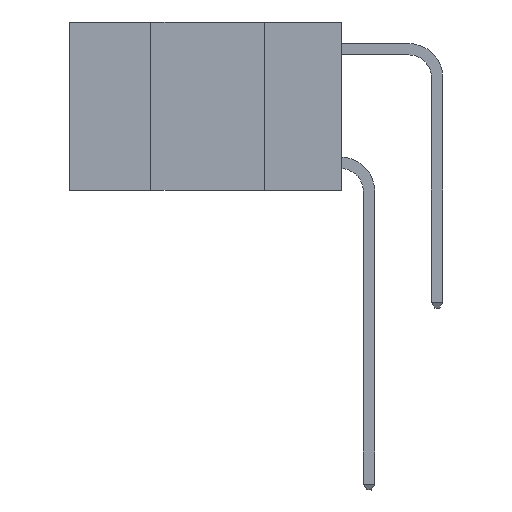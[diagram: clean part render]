
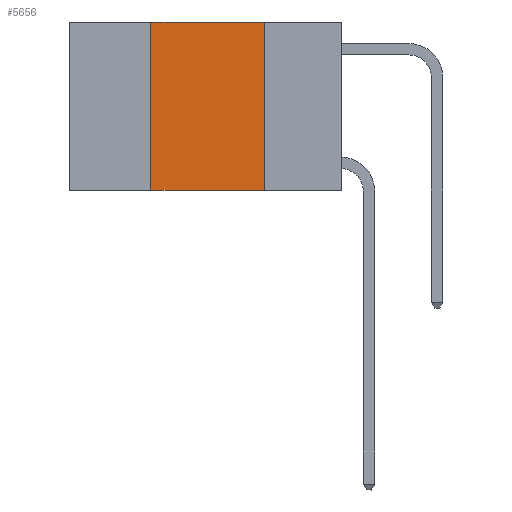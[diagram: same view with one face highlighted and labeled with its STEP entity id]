
A CAD part, left-side view. The second image highlights one B-rep face of the part: STEP entity #5656.
In plain terms, the highlighted planar face has unit normal (-1, 0, 0).
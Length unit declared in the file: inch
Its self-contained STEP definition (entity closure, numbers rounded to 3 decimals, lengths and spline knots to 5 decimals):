
#316 = FACE_OUTER_BOUND ( 'NONE', #9335, .T. ) ;
#347 = VECTOR ( 'NONE', #8103, 39.37008 ) ;
#1225 = LINE ( 'NONE', #9011, #8195 ) ;
#1797 = VECTOR ( 'NONE', #2323, 39.37008 ) ;
#2323 = DIRECTION ( 'NONE',  ( 0., 0., -1. ) ) ;
#2434 = VERTEX_POINT ( 'NONE', #15414 ) ;
#3010 = DIRECTION ( 'NONE',  ( 0., 0., -1. ) ) ;
#3674 = CARTESIAN_POINT ( 'NONE',  ( 0., 0.42, 0. ) ) ;
#3775 = EDGE_CURVE ( 'NONE', #13222, #13235, #6235, .T. ) ;
#4371 = ORIENTED_EDGE ( 'NONE', *, *, #16901, .F. ) ;
#4455 = PLANE ( 'NONE',  #18469 ) ;
#4460 = CARTESIAN_POINT ( 'NONE',  ( 0., 0.42, -0.37 ) ) ;
#5656 = ADVANCED_FACE ( 'NONE', ( #316 ), #4455, .F. ) ;
#6161 = LINE ( 'NONE', #6517, #10000 ) ;
#6235 = LINE ( 'NONE', #9651, #1797 ) ;
#6451 = EDGE_CURVE ( 'NONE', #18602, #13235, #6161, .T. ) ;
#6517 = CARTESIAN_POINT ( 'NONE',  ( 0., 0.6, -0.37 ) ) ;
#6994 = EDGE_CURVE ( 'NONE', #2434, #13222, #1225, .T. ) ;
#7396 = CARTESIAN_POINT ( 'NONE',  ( 0., 0.6, 0. ) ) ;
#8103 = DIRECTION ( 'NONE',  ( 0., 0., 1. ) ) ;
#8195 = VECTOR ( 'NONE', #10453, 39.37008 ) ;
#8261 = ORIENTED_EDGE ( 'NONE', *, *, #6451, .T. ) ;
#8407 = CARTESIAN_POINT ( 'NONE',  ( 0., 0.17, -0.37 ) ) ;
#9011 = CARTESIAN_POINT ( 'NONE',  ( 0., 0.6, 0. ) ) ;
#9335 = EDGE_LOOP ( 'NONE', ( #18921, #11632, #4371, #8261 ) ) ;
#9651 = CARTESIAN_POINT ( 'NONE',  ( 0., 0.17, 0. ) ) ;
#10000 = VECTOR ( 'NONE', #15199, 39.37008 ) ;
#10453 = DIRECTION ( 'NONE',  ( 0., -1., 0. ) ) ;
#11632 = ORIENTED_EDGE ( 'NONE', *, *, #6994, .F. ) ;
#11740 = DIRECTION ( 'NONE',  ( 1., 0., 0. ) ) ;
#13222 = VERTEX_POINT ( 'NONE', #18512 ) ;
#13235 = VERTEX_POINT ( 'NONE', #8407 ) ;
#15199 = DIRECTION ( 'NONE',  ( 0., -1., 0. ) ) ;
#15414 = CARTESIAN_POINT ( 'NONE',  ( 0., 0.42, 0. ) ) ;
#16432 = LINE ( 'NONE', #3674, #347 ) ;
#16901 = EDGE_CURVE ( 'NONE', #18602, #2434, #16432, .T. ) ;
#18469 = AXIS2_PLACEMENT_3D ( 'NONE', #7396, #11740, #3010 ) ;
#18512 = CARTESIAN_POINT ( 'NONE',  ( 0., 0.17, 0. ) ) ;
#18602 = VERTEX_POINT ( 'NONE', #4460 ) ;
#18921 = ORIENTED_EDGE ( 'NONE', *, *, #3775, .F. ) ;
